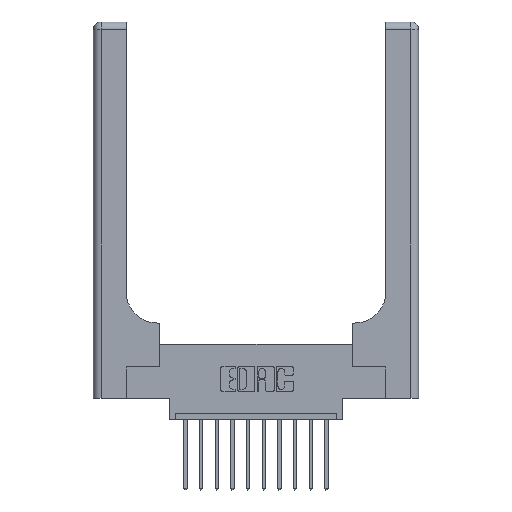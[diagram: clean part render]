
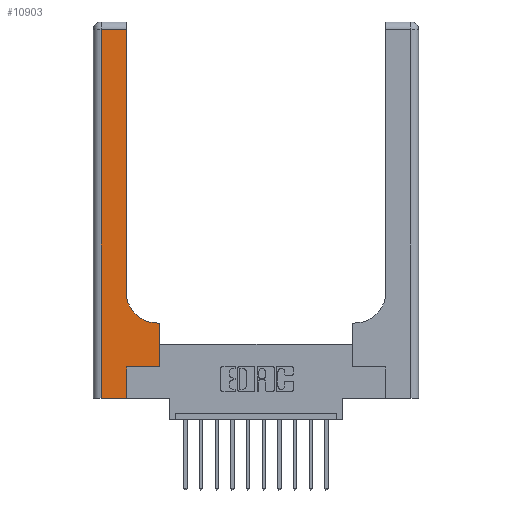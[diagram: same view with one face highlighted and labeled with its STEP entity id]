
A CAD part, top view. The second image highlights one B-rep face of the part: STEP entity #10903.
In plain terms, the highlighted planar face has unit normal (0, 0, 1).
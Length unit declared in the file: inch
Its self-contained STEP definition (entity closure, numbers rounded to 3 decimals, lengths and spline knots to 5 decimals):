
#74 = VECTOR ( 'NONE', #893, 39.37008 ) ;
#146 = AXIS2_PLACEMENT_3D ( 'NONE', #248, #5446, #4207 ) ;
#248 = CARTESIAN_POINT ( 'NONE',  ( 0., 3., 0.37 ) ) ;
#608 = LINE ( 'NONE', #15677, #10353 ) ;
#893 = DIRECTION ( 'NONE',  ( -1., 0., 0. ) ) ;
#1154 = ORIENTED_EDGE ( 'NONE', *, *, #2424, .T. ) ;
#1186 = VECTOR ( 'NONE', #4570, 39.37008 ) ;
#1329 = VERTEX_POINT ( 'NONE', #6153 ) ;
#1366 = LINE ( 'NONE', #16090, #2289 ) ;
#1537 = EDGE_CURVE ( 'NONE', #12228, #6299, #1894, .T. ) ;
#1894 = LINE ( 'NONE', #13007, #9915 ) ;
#2176 = EDGE_CURVE ( 'NONE', #12610, #2470, #1366, .T. ) ;
#2289 = VECTOR ( 'NONE', #4844, 39.37008 ) ;
#2424 = EDGE_CURVE ( 'NONE', #11003, #14329, #15832, .T. ) ;
#2470 = VERTEX_POINT ( 'NONE', #12131 ) ;
#2488 = CARTESIAN_POINT ( 'NONE',  ( 0.26, 2.94, 0.37 ) ) ;
#3082 = CIRCLE ( 'NONE', #13076, 0.25 ) ;
#3248 = DIRECTION ( 'NONE',  ( 0., 1., 0. ) ) ;
#3299 = CARTESIAN_POINT ( 'NONE',  ( 0.26, 0.6, 0.37 ) ) ;
#3548 = EDGE_CURVE ( 'NONE', #1329, #11003, #608, .T. ) ;
#4207 = DIRECTION ( 'NONE',  ( -1., 0., 0. ) ) ;
#4374 = VECTOR ( 'NONE', #8220, 39.37008 ) ;
#4415 = LINE ( 'NONE', #13510, #1186 ) ;
#4570 = DIRECTION ( 'NONE',  ( -1., 0., 0. ) ) ;
#4844 = DIRECTION ( 'NONE',  ( 0., 1., 0. ) ) ;
#5347 = LINE ( 'NONE', #15687, #4374 ) ;
#5446 = DIRECTION ( 'NONE',  ( 0., 0., -1. ) ) ;
#5497 = VERTEX_POINT ( 'NONE', #12396 ) ;
#5504 = DIRECTION ( 'NONE',  ( 1., 0., 0. ) ) ;
#5627 = ORIENTED_EDGE ( 'NONE', *, *, #2176, .T. ) ;
#5817 = EDGE_CURVE ( 'NONE', #14329, #12610, #5827, .T. ) ;
#5827 = LINE ( 'NONE', #7136, #14400 ) ;
#5894 = EDGE_LOOP ( 'NONE', ( #8743, #14742, #14636, #15625, #1154, #9494, #5627, #11077, #11362 ) ) ;
#6153 = CARTESIAN_POINT ( 'NONE',  ( 0.06, 0., 0.37 ) ) ;
#6176 = EDGE_CURVE ( 'NONE', #6299, #5497, #4415, .T. ) ;
#6299 = VERTEX_POINT ( 'NONE', #2488 ) ;
#6782 = EDGE_CURVE ( 'NONE', #5497, #1329, #5347, .T. ) ;
#7136 = CARTESIAN_POINT ( 'NONE',  ( 0.265, 0.25, 0.37 ) ) ;
#7564 = CARTESIAN_POINT ( 'NONE',  ( 0.51, 0.6, 0.37 ) ) ;
#7662 = DIRECTION ( 'NONE',  ( 1., 0., 0. ) ) ;
#7828 = FACE_OUTER_BOUND ( 'NONE', #5894, .T. ) ;
#7951 = EDGE_CURVE ( 'NONE', #2470, #11272, #13495, .T. ) ;
#8220 = DIRECTION ( 'NONE',  ( 0., -1., 0. ) ) ;
#8401 = CARTESIAN_POINT ( 'NONE',  ( 0.26, 0.85, 0.37 ) ) ;
#8743 = ORIENTED_EDGE ( 'NONE', *, *, #1537, .T. ) ;
#9494 = ORIENTED_EDGE ( 'NONE', *, *, #5817, .T. ) ;
#9915 = VECTOR ( 'NONE', #14322, 39.37008 ) ;
#10353 = VECTOR ( 'NONE', #5504, 39.37008 ) ;
#10834 = DIRECTION ( 'NONE',  ( 1., 0., 0. ) ) ;
#10903 = ADVANCED_FACE ( 'NONE', ( #7828 ), #11523, .F. ) ;
#11003 = VERTEX_POINT ( 'NONE', #14478 ) ;
#11077 = ORIENTED_EDGE ( 'NONE', *, *, #7951, .T. ) ;
#11272 = VERTEX_POINT ( 'NONE', #7564 ) ;
#11362 = ORIENTED_EDGE ( 'NONE', *, *, #12088, .T. ) ;
#11523 = PLANE ( 'NONE',  #146 ) ;
#11796 = CARTESIAN_POINT ( 'NONE',  ( 0.265, 0.25, 0.37 ) ) ;
#11999 = VECTOR ( 'NONE', #3248, 39.37008 ) ;
#12088 = EDGE_CURVE ( 'NONE', #11272, #12228, #3082, .T. ) ;
#12131 = CARTESIAN_POINT ( 'NONE',  ( 0.528, 0.6, 0.37 ) ) ;
#12228 = VERTEX_POINT ( 'NONE', #8401 ) ;
#12396 = CARTESIAN_POINT ( 'NONE',  ( 0.06, 2.94, 0.37 ) ) ;
#12610 = VERTEX_POINT ( 'NONE', #16149 ) ;
#12841 = CARTESIAN_POINT ( 'NONE',  ( 0.51, 0.85, 0.37 ) ) ;
#13007 = CARTESIAN_POINT ( 'NONE',  ( 0.26, 3., 0.37 ) ) ;
#13076 = AXIS2_PLACEMENT_3D ( 'NONE', #12841, #15382, #7662 ) ;
#13495 = LINE ( 'NONE', #3299, #74 ) ;
#13510 = CARTESIAN_POINT ( 'NONE',  ( 0., 2.94, 0.37 ) ) ;
#14322 = DIRECTION ( 'NONE',  ( 0., 1., 0. ) ) ;
#14329 = VERTEX_POINT ( 'NONE', #11796 ) ;
#14400 = VECTOR ( 'NONE', #10834, 39.37008 ) ;
#14478 = CARTESIAN_POINT ( 'NONE',  ( 0.265, 0., 0.37 ) ) ;
#14527 = CARTESIAN_POINT ( 'NONE',  ( 0.265, 0., 0.37 ) ) ;
#14636 = ORIENTED_EDGE ( 'NONE', *, *, #6782, .T. ) ;
#14742 = ORIENTED_EDGE ( 'NONE', *, *, #6176, .T. ) ;
#15382 = DIRECTION ( 'NONE',  ( 0., 0., -1. ) ) ;
#15625 = ORIENTED_EDGE ( 'NONE', *, *, #3548, .T. ) ;
#15677 = CARTESIAN_POINT ( 'NONE',  ( 0., 0., 0.37 ) ) ;
#15687 = CARTESIAN_POINT ( 'NONE',  ( 0.06, 3., 0.37 ) ) ;
#15832 = LINE ( 'NONE', #14527, #11999 ) ;
#16090 = CARTESIAN_POINT ( 'NONE',  ( 0.528, 0.25, 0.37 ) ) ;
#16149 = CARTESIAN_POINT ( 'NONE',  ( 0.528, 0.25, 0.37 ) ) ;
